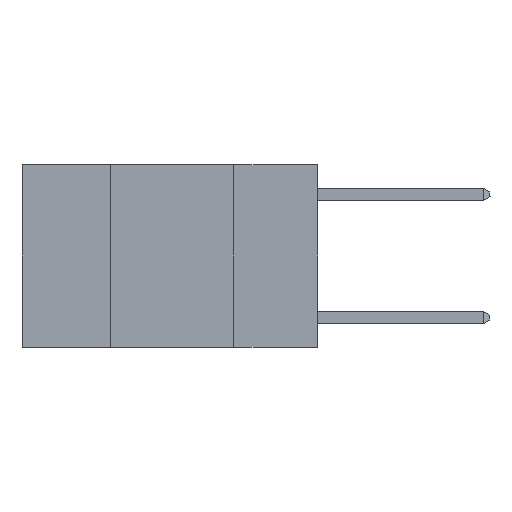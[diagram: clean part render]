
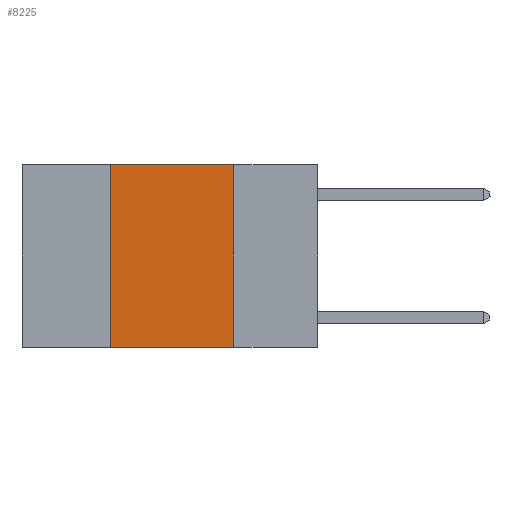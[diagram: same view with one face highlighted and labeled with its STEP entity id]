
A CAD part, left-side view. The second image highlights one B-rep face of the part: STEP entity #8225.
In plain terms, the highlighted planar face has unit normal (-1, 0, 0).
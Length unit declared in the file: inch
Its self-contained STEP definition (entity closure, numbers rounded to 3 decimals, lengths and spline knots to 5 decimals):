
#648 = CARTESIAN_POINT ( 'NONE',  ( 0., 0.6, -0.37 ) ) ;
#958 = ORIENTED_EDGE ( 'NONE', *, *, #9780, .F. ) ;
#964 = CARTESIAN_POINT ( 'NONE',  ( 0., 0.42, -0.37 ) ) ;
#1203 = DIRECTION ( 'NONE',  ( 1., 0., 0. ) ) ;
#1355 = LINE ( 'NONE', #16951, #4964 ) ;
#1568 = ORIENTED_EDGE ( 'NONE', *, *, #5625, .T. ) ;
#1619 = DIRECTION ( 'NONE',  ( 0., 0., -1. ) ) ;
#2607 = CARTESIAN_POINT ( 'NONE',  ( 0., 0.17, 0. ) ) ;
#3503 = CARTESIAN_POINT ( 'NONE',  ( 0., 0.6, 0. ) ) ;
#3949 = VERTEX_POINT ( 'NONE', #964 ) ;
#4254 = LINE ( 'NONE', #648, #14429 ) ;
#4852 = DIRECTION ( 'NONE',  ( 0., -1., 0. ) ) ;
#4964 = VECTOR ( 'NONE', #9099, 39.37008 ) ;
#5345 = VERTEX_POINT ( 'NONE', #9556 ) ;
#5574 = AXIS2_PLACEMENT_3D ( 'NONE', #17121, #1203, #10599 ) ;
#5625 = EDGE_CURVE ( 'NONE', #3949, #12179, #4254, .T. ) ;
#6737 = LINE ( 'NONE', #3503, #13370 ) ;
#7601 = EDGE_CURVE ( 'NONE', #5345, #14190, #6737, .T. ) ;
#7944 = PLANE ( 'NONE',  #5574 ) ;
#8225 = ADVANCED_FACE ( 'NONE', ( #14374 ), #7944, .F. ) ;
#9099 = DIRECTION ( 'NONE',  ( 0., 0., 1. ) ) ;
#9556 = CARTESIAN_POINT ( 'NONE',  ( 0., 0.42, 0. ) ) ;
#9780 = EDGE_CURVE ( 'NONE', #14190, #12179, #10053, .T. ) ;
#9905 = EDGE_LOOP ( 'NONE', ( #958, #13897, #11549, #1568 ) ) ;
#10053 = LINE ( 'NONE', #14923, #13558 ) ;
#10599 = DIRECTION ( 'NONE',  ( 0., 0., -1. ) ) ;
#11402 = EDGE_CURVE ( 'NONE', #3949, #5345, #1355, .T. ) ;
#11549 = ORIENTED_EDGE ( 'NONE', *, *, #11402, .F. ) ;
#12179 = VERTEX_POINT ( 'NONE', #13242 ) ;
#13242 = CARTESIAN_POINT ( 'NONE',  ( 0., 0.17, -0.37 ) ) ;
#13370 = VECTOR ( 'NONE', #4852, 39.37008 ) ;
#13558 = VECTOR ( 'NONE', #1619, 39.37008 ) ;
#13897 = ORIENTED_EDGE ( 'NONE', *, *, #7601, .F. ) ;
#14190 = VERTEX_POINT ( 'NONE', #2607 ) ;
#14374 = FACE_OUTER_BOUND ( 'NONE', #9905, .T. ) ;
#14429 = VECTOR ( 'NONE', #15352, 39.37008 ) ;
#14923 = CARTESIAN_POINT ( 'NONE',  ( 0., 0.17, 0. ) ) ;
#15352 = DIRECTION ( 'NONE',  ( 0., -1., 0. ) ) ;
#16951 = CARTESIAN_POINT ( 'NONE',  ( 0., 0.42, 0. ) ) ;
#17121 = CARTESIAN_POINT ( 'NONE',  ( 0., 0.6, 0. ) ) ;
